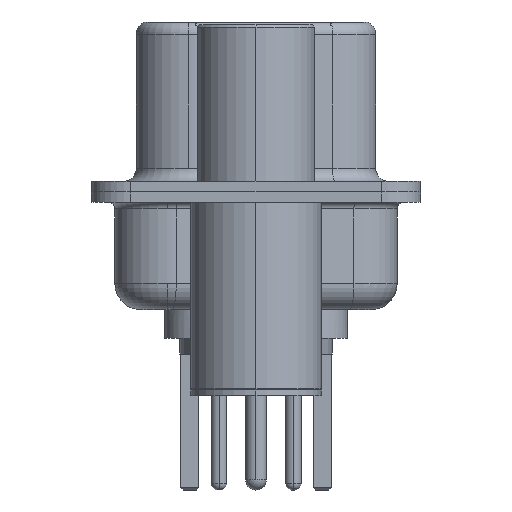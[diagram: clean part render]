
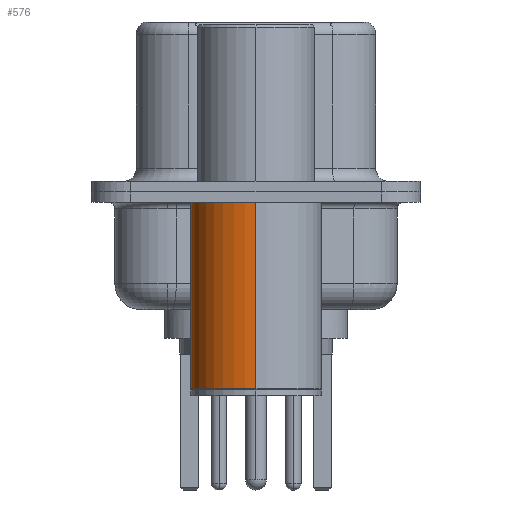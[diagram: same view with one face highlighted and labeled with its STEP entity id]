
A CAD part, left-side view. The second image highlights one B-rep face of the part: STEP entity #576.
In plain terms, the highlighted cylindrical face has radius 2.5 mm (diameter 5 mm), a partial arc.
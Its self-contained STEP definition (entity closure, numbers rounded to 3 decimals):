
#55 = VERTEX_POINT ( 'NONE', #10667 ) ;
#61 = LINE ( 'NONE', #4769, #16440 ) ;
#576 = ADVANCED_FACE ( 'NONE', ( #18607 ), #828, .T. ) ;
#828 = CYLINDRICAL_SURFACE ( 'NONE', #19769, 2.5 ) ;
#1151 = CARTESIAN_POINT ( 'NONE',  ( 0., 0., -0.4 ) ) ;
#1162 = ORIENTED_EDGE ( 'NONE', *, *, #14314, .F. ) ;
#1739 = ORIENTED_EDGE ( 'NONE', *, *, #14524, .F. ) ;
#2232 = CARTESIAN_POINT ( 'NONE',  ( 0., 0., -7.525 ) ) ;
#3235 = DIRECTION ( 'NONE',  ( 1., 0., 0. ) ) ;
#4280 = CARTESIAN_POINT ( 'NONE',  ( -2.5, 0., -0.4 ) ) ;
#4281 = DIRECTION ( 'NONE',  ( 1., 0., 0. ) ) ;
#4769 = CARTESIAN_POINT ( 'NONE',  ( -2.5, 0., 0.581 ) ) ;
#5038 = CIRCLE ( 'NONE', #21516, 2.5 ) ;
#5216 = AXIS2_PLACEMENT_3D ( 'NONE', #2232, #17184, #4281 ) ;
#5756 = EDGE_LOOP ( 'NONE', ( #26994, #22030, #1162, #1739 ) ) ;
#7154 = VERTEX_POINT ( 'NONE', #4280 ) ;
#10420 = CARTESIAN_POINT ( 'NONE',  ( 2.5, 0., 0.581 ) ) ;
#10667 = CARTESIAN_POINT ( 'NONE',  ( -2.5, 0., -7.525 ) ) ;
#11243 = DIRECTION ( 'NONE',  ( 0., 0., 1. ) ) ;
#12275 = CARTESIAN_POINT ( 'NONE',  ( 2.5, 0., -7.525 ) ) ;
#13275 = EDGE_CURVE ( 'NONE', #55, #7154, #61, .T. ) ;
#13806 = EDGE_CURVE ( 'NONE', #14460, #55, #24164, .T. ) ;
#14314 = EDGE_CURVE ( 'NONE', #18189, #7154, #5038, .T. ) ;
#14460 = VERTEX_POINT ( 'NONE', #12275 ) ;
#14524 = EDGE_CURVE ( 'NONE', #14460, #18189, #18936, .T. ) ;
#16080 = DIRECTION ( 'NONE',  ( 0., 0., 1. ) ) ;
#16258 = DIRECTION ( 'NONE',  ( 1., 0., 0. ) ) ;
#16416 = CARTESIAN_POINT ( 'NONE',  ( 2.5, 0., -0.4 ) ) ;
#16440 = VECTOR ( 'NONE', #11243, 1000. ) ;
#16782 = CARTESIAN_POINT ( 'NONE',  ( 0., 0., 0.581 ) ) ;
#16845 = VECTOR ( 'NONE', #23297, 1000. ) ;
#17078 = DIRECTION ( 'NONE',  ( 0., 0., 1. ) ) ;
#17184 = DIRECTION ( 'NONE',  ( 0., 0., 1. ) ) ;
#18189 = VERTEX_POINT ( 'NONE', #16416 ) ;
#18607 = FACE_OUTER_BOUND ( 'NONE', #5756, .T. ) ;
#18936 = LINE ( 'NONE', #10420, #16845 ) ;
#19769 = AXIS2_PLACEMENT_3D ( 'NONE', #16782, #17078, #16258 ) ;
#21516 = AXIS2_PLACEMENT_3D ( 'NONE', #1151, #16080, #3235 ) ;
#22030 = ORIENTED_EDGE ( 'NONE', *, *, #13275, .T. ) ;
#23297 = DIRECTION ( 'NONE',  ( 0., 0., 1. ) ) ;
#24164 = CIRCLE ( 'NONE', #5216, 2.5 ) ;
#26994 = ORIENTED_EDGE ( 'NONE', *, *, #13806, .T. ) ;
